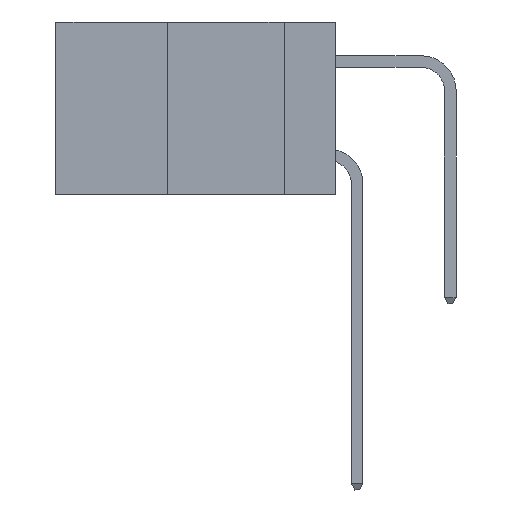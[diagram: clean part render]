
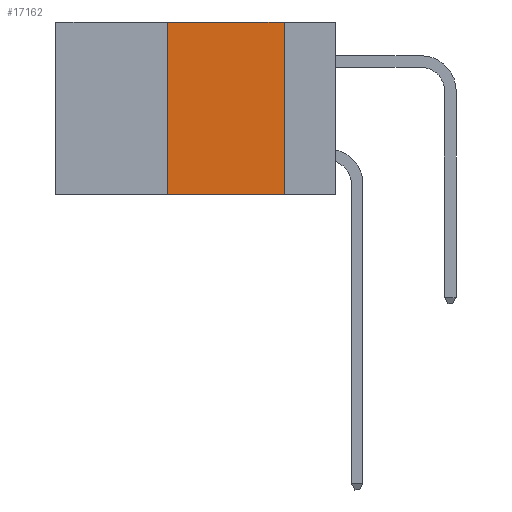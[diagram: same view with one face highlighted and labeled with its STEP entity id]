
A CAD part, left-side view. The second image highlights one B-rep face of the part: STEP entity #17162.
In plain terms, the highlighted planar face has unit normal (-1, 0, 0).
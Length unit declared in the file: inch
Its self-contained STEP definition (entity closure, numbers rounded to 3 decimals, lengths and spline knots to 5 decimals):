
#237 = VECTOR ( 'NONE', #20216, 39.37008 ) ;
#1303 = ORIENTED_EDGE ( 'NONE', *, *, #10417, .F. ) ;
#1714 = LINE ( 'NONE', #12664, #5862 ) ;
#2849 = EDGE_CURVE ( 'NONE', #18861, #17172, #12478, .T. ) ;
#3213 = EDGE_LOOP ( 'NONE', ( #1303, #24195, #21240, #9355 ) ) ;
#4007 = VERTEX_POINT ( 'NONE', #24266 ) ;
#5862 = VECTOR ( 'NONE', #19274, 39.37008 ) ;
#7923 = DIRECTION ( 'NONE',  ( 0., -1., 0. ) ) ;
#9355 = ORIENTED_EDGE ( 'NONE', *, *, #2849, .T. ) ;
#10417 = EDGE_CURVE ( 'NONE', #12195, #17172, #16721, .T. ) ;
#11030 = CARTESIAN_POINT ( 'NONE',  ( 0., 0.11, -0.37 ) ) ;
#11304 = PLANE ( 'NONE',  #25802 ) ;
#12195 = VERTEX_POINT ( 'NONE', #20612 ) ;
#12478 = LINE ( 'NONE', #18819, #20592 ) ;
#12664 = CARTESIAN_POINT ( 'NONE',  ( 0., 0.36, 0. ) ) ;
#13405 = DIRECTION ( 'NONE',  ( 1., 0., 0. ) ) ;
#13884 = CARTESIAN_POINT ( 'NONE',  ( 0., 0.6, 0. ) ) ;
#14311 = EDGE_CURVE ( 'NONE', #4007, #12195, #20857, .T. ) ;
#14640 = DIRECTION ( 'NONE',  ( 0., -1., 0. ) ) ;
#16721 = LINE ( 'NONE', #17830, #237 ) ;
#17162 = ADVANCED_FACE ( 'NONE', ( #20367 ), #11304, .F. ) ;
#17172 = VERTEX_POINT ( 'NONE', #11030 ) ;
#17830 = CARTESIAN_POINT ( 'NONE',  ( 0., 0.11, 0. ) ) ;
#18819 = CARTESIAN_POINT ( 'NONE',  ( 0., 0.6, -0.37 ) ) ;
#18861 = VERTEX_POINT ( 'NONE', #23849 ) ;
#19274 = DIRECTION ( 'NONE',  ( 0., 0., 1. ) ) ;
#19289 = DIRECTION ( 'NONE',  ( 0., 0., -1. ) ) ;
#20216 = DIRECTION ( 'NONE',  ( 0., 0., -1. ) ) ;
#20367 = FACE_OUTER_BOUND ( 'NONE', #3213, .T. ) ;
#20592 = VECTOR ( 'NONE', #14640, 39.37008 ) ;
#20612 = CARTESIAN_POINT ( 'NONE',  ( 0., 0.11, 0. ) ) ;
#20857 = LINE ( 'NONE', #13884, #24488 ) ;
#21240 = ORIENTED_EDGE ( 'NONE', *, *, #25221, .F. ) ;
#23578 = CARTESIAN_POINT ( 'NONE',  ( 0., 0.6, 0. ) ) ;
#23849 = CARTESIAN_POINT ( 'NONE',  ( 0., 0.36, -0.37 ) ) ;
#24195 = ORIENTED_EDGE ( 'NONE', *, *, #14311, .F. ) ;
#24266 = CARTESIAN_POINT ( 'NONE',  ( 0., 0.36, 0. ) ) ;
#24488 = VECTOR ( 'NONE', #7923, 39.37008 ) ;
#25221 = EDGE_CURVE ( 'NONE', #18861, #4007, #1714, .T. ) ;
#25802 = AXIS2_PLACEMENT_3D ( 'NONE', #23578, #13405, #19289 ) ;
